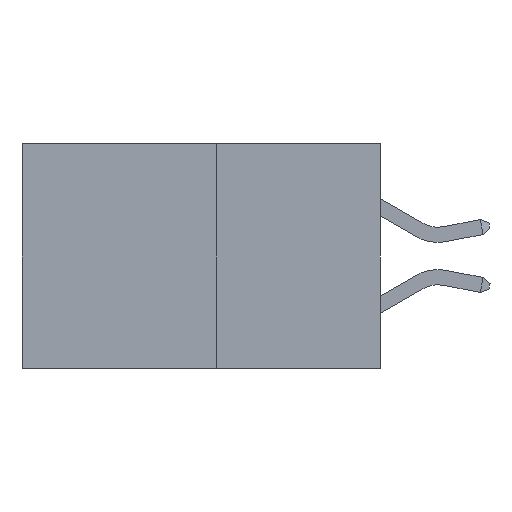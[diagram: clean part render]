
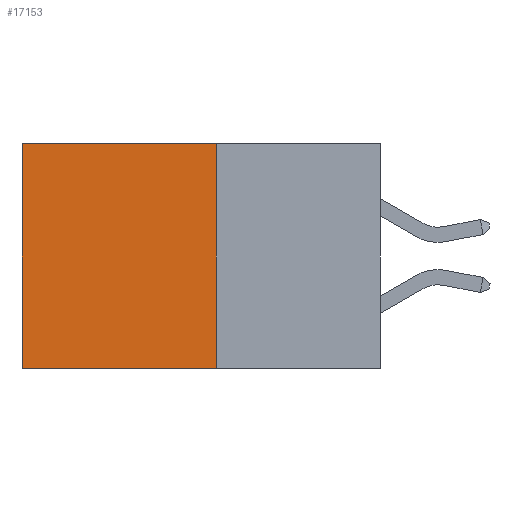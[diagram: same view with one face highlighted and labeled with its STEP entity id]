
A CAD part, left-side view. The second image highlights one B-rep face of the part: STEP entity #17153.
In plain terms, the highlighted planar face has unit normal (-1, 0, 0).
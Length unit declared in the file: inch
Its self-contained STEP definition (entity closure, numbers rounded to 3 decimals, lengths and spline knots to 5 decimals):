
#444 = EDGE_CURVE ( 'NONE', #16342, #17720, #10405, .T. ) ;
#890 = VERTEX_POINT ( 'NONE', #10701 ) ;
#919 = VECTOR ( 'NONE', #23334, 39.37008 ) ;
#1622 = VERTEX_POINT ( 'NONE', #5360 ) ;
#1798 = DIRECTION ( 'NONE',  ( 0., 0., -1. ) ) ;
#3090 = EDGE_CURVE ( 'NONE', #890, #17720, #15699, .T. ) ;
#5360 = CARTESIAN_POINT ( 'NONE',  ( 0.277, 0.27, 0. ) ) ;
#5549 = VECTOR ( 'NONE', #19975, 39.37008 ) ;
#6004 = ORIENTED_EDGE ( 'NONE', *, *, #17016, .F. ) ;
#6713 = CARTESIAN_POINT ( 'NONE',  ( 0.277, 0.27, -0.37 ) ) ;
#7358 = EDGE_LOOP ( 'NONE', ( #15746, #23013, #6004, #22995 ) ) ;
#8692 = LINE ( 'NONE', #17980, #18229 ) ;
#9334 = PLANE ( 'NONE',  #11721 ) ;
#10043 = VECTOR ( 'NONE', #12773, 39.37008 ) ;
#10405 = LINE ( 'NONE', #6713, #919 ) ;
#10701 = CARTESIAN_POINT ( 'NONE',  ( 0.277, 0.59, 0. ) ) ;
#10848 = CARTESIAN_POINT ( 'NONE',  ( 0.277, 0.27, -0.37 ) ) ;
#11542 = FACE_OUTER_BOUND ( 'NONE', #7358, .T. ) ;
#11721 = AXIS2_PLACEMENT_3D ( 'NONE', #24509, #13195, #1798 ) ;
#12773 = DIRECTION ( 'NONE',  ( 0., 0., -1. ) ) ;
#13195 = DIRECTION ( 'NONE',  ( 1., 0., 0. ) ) ;
#15699 = LINE ( 'NONE', #20038, #5549 ) ;
#15746 = ORIENTED_EDGE ( 'NONE', *, *, #3090, .T. ) ;
#16342 = VERTEX_POINT ( 'NONE', #18529 ) ;
#17016 = EDGE_CURVE ( 'NONE', #1622, #16342, #20737, .T. ) ;
#17153 = ADVANCED_FACE ( 'NONE', ( #11542 ), #9334, .F. ) ;
#17720 = VERTEX_POINT ( 'NONE', #22339 ) ;
#17980 = CARTESIAN_POINT ( 'NONE',  ( 0.277, 0.27, 0. ) ) ;
#18229 = VECTOR ( 'NONE', #19852, 39.37008 ) ;
#18529 = CARTESIAN_POINT ( 'NONE',  ( 0.277, 0.27, -0.37 ) ) ;
#19852 = DIRECTION ( 'NONE',  ( 0., 1., 0. ) ) ;
#19975 = DIRECTION ( 'NONE',  ( 0., 0., -1. ) ) ;
#20038 = CARTESIAN_POINT ( 'NONE',  ( 0.277, 0.59, -0.37 ) ) ;
#20737 = LINE ( 'NONE', #10848, #10043 ) ;
#22339 = CARTESIAN_POINT ( 'NONE',  ( 0.277, 0.59, -0.37 ) ) ;
#22995 = ORIENTED_EDGE ( 'NONE', *, *, #23271, .T. ) ;
#23013 = ORIENTED_EDGE ( 'NONE', *, *, #444, .F. ) ;
#23271 = EDGE_CURVE ( 'NONE', #1622, #890, #8692, .T. ) ;
#23334 = DIRECTION ( 'NONE',  ( 0., 1., 0. ) ) ;
#24509 = CARTESIAN_POINT ( 'NONE',  ( 0.277, 0.27, -0.37 ) ) ;
